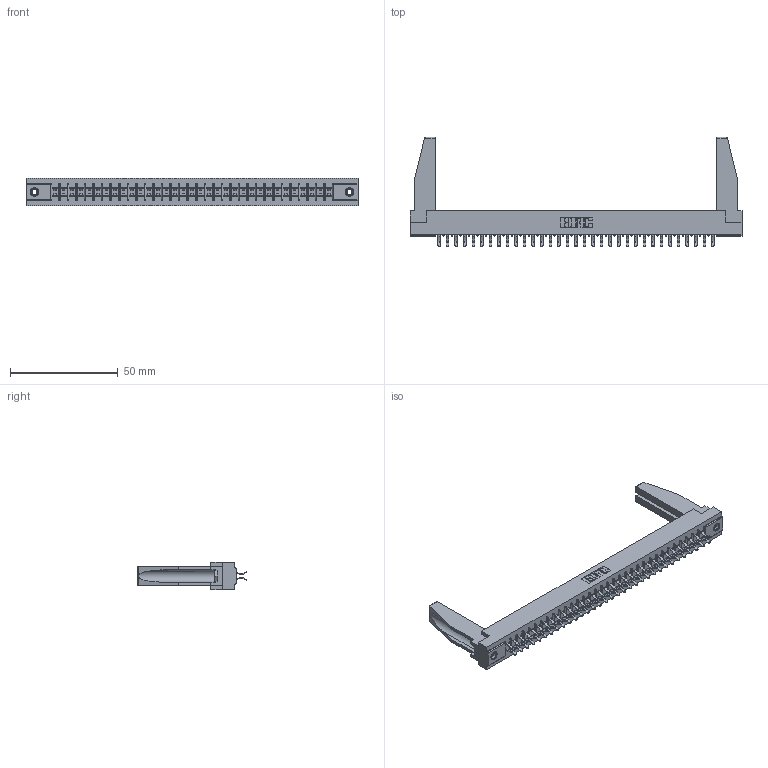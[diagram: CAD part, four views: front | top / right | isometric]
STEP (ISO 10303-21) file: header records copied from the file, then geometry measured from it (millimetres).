
FILE_DESCRIPTION (( 'STEP AP203' ), '1' );
FILE_NAME ('315-066-556-278.STEP', '2019-09-10T21:00:48', ( '' ), ( '' ), 'SwSTEP 2.0', 'SolidWorks 2016', '' );
FILE_SCHEMA (( 'CONFIG_CONTROL_DESIGN' ));
Length unit declared in the file: inch
Products named in the file (5): 305 Part_.156 Dia; 305-290-001_556; 307-220-078; 345-250-001_345-250-001-102; 315-066-556-278
Assembly tree (71 placements, depth 2):
  315-066-556-278
    305 Part_.156 Dia
    305-290-001_556  x66
    345-250-001_345-250-001-102  x2
    307-220-078  x2
Bounding box: 153.77 x 50.67 x 12.7 mm (x, y, z)
Volume: 19974.5 mm3; surface area: 23966.1 mm2
Topology: 71 solids, 71 shells, 3942 faces, 11305 edges, 7350 vertices
Faces by surface type: plane 2198, cylinder 1596, sphere 132, cone 12, torus 4
Entity records: 39487 total; most frequent: CARTESIAN_POINT 6543, ORIENTED_EDGE 6452, DIRECTION 6298, EDGE_CURVE 3226, LINE 2592, VECTOR 2592, VERTEX_POINT 2056, AXIS2_PLACEMENT_3D 1853
